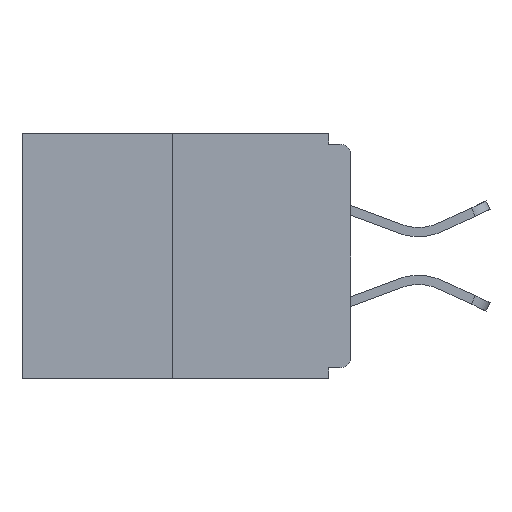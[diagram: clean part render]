
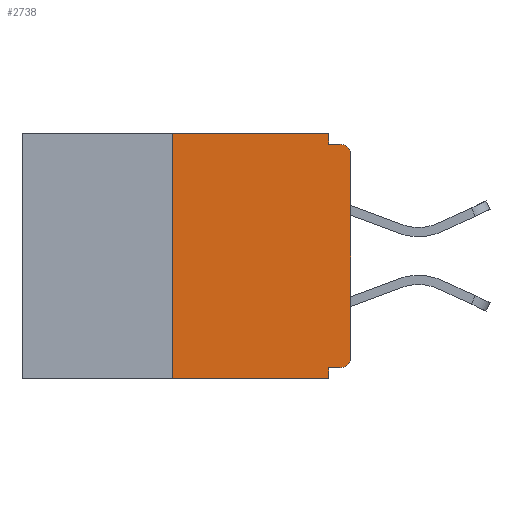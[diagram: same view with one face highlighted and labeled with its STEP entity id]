
A CAD part, left-side view. The second image highlights one B-rep face of the part: STEP entity #2738.
In plain terms, the highlighted planar face has unit normal (-1, 0, 0).
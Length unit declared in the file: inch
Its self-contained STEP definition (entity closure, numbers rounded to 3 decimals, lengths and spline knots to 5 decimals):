
#90 = DIRECTION ( 'NONE',  ( 0., 0., -1. ) ) ;
#414 = VECTOR ( 'NONE', #5295, 39.37008 ) ;
#443 = CARTESIAN_POINT ( 'NONE',  ( 0., 0.031, -0.015 ) ) ;
#765 = AXIS2_PLACEMENT_3D ( 'NONE', #9386, #5205, #12237 ) ;
#822 = CIRCLE ( 'NONE', #15565, 0.015 ) ;
#994 = CARTESIAN_POINT ( 'NONE',  ( 0., 0., -0.015 ) ) ;
#1052 = DIRECTION ( 'NONE',  ( 0., -1., 0. ) ) ;
#1104 = DIRECTION ( 'NONE',  ( 0., 1., 0. ) ) ;
#1154 = DIRECTION ( 'NONE',  ( 0., 0., 1. ) ) ;
#1769 = LINE ( 'NONE', #17970, #414 ) ;
#1825 = CIRCLE ( 'NONE', #765, 0.015 ) ;
#1953 = DIRECTION ( 'NONE',  ( 0., -1., 0. ) ) ;
#2083 = DIRECTION ( 'NONE',  ( 0., 0., -1. ) ) ;
#2545 = LINE ( 'NONE', #9125, #6310 ) ;
#2627 = LINE ( 'NONE', #17397, #12072 ) ;
#2664 = EDGE_CURVE ( 'NONE', #4280, #16776, #12251, .T. ) ;
#2697 = CARTESIAN_POINT ( 'NONE',  ( 0., 0.25, 0. ) ) ;
#2738 = ADVANCED_FACE ( 'NONE', ( #11829 ), #7510, .F. ) ;
#2756 = EDGE_CURVE ( 'NONE', #16776, #17188, #14868, .T. ) ;
#3808 = CARTESIAN_POINT ( 'NONE',  ( 0., 0., 0. ) ) ;
#4280 = VERTEX_POINT ( 'NONE', #15031 ) ;
#4948 = CARTESIAN_POINT ( 'NONE',  ( 0., 0.015, -0.015 ) ) ;
#5205 = DIRECTION ( 'NONE',  ( -1., 0., 0. ) ) ;
#5295 = DIRECTION ( 'NONE',  ( 0., -1., 0. ) ) ;
#5368 = ORIENTED_EDGE ( 'NONE', *, *, #13548, .F. ) ;
#5560 = CARTESIAN_POINT ( 'NONE',  ( 0., 0.25, -0.343 ) ) ;
#5586 = EDGE_LOOP ( 'NONE', ( #10900, #16993, #12227, #5658, #12666, #16436, #12895, #8664, #8403, #5368 ) ) ;
#5616 = VECTOR ( 'NONE', #6589, 39.37008 ) ;
#5658 = ORIENTED_EDGE ( 'NONE', *, *, #2756, .F. ) ;
#5759 = CARTESIAN_POINT ( 'NONE',  ( 0., 0.015, -0.313 ) ) ;
#6137 = EDGE_CURVE ( 'NONE', #11854, #13108, #1825, .T. ) ;
#6310 = VECTOR ( 'NONE', #2083, 39.37008 ) ;
#6589 = DIRECTION ( 'NONE',  ( 0., 0., 1. ) ) ;
#6967 = VECTOR ( 'NONE', #1104, 39.37008 ) ;
#7136 = VERTEX_POINT ( 'NONE', #443 ) ;
#7269 = DIRECTION ( 'NONE',  ( 0., 0., -1. ) ) ;
#7510 = PLANE ( 'NONE',  #13661 ) ;
#8403 = ORIENTED_EDGE ( 'NONE', *, *, #16284, .F. ) ;
#8664 = ORIENTED_EDGE ( 'NONE', *, *, #6137, .T. ) ;
#9125 = CARTESIAN_POINT ( 'NONE',  ( 0., 0.031, 0. ) ) ;
#9386 = CARTESIAN_POINT ( 'NONE',  ( 0., 0.015, -0.03 ) ) ;
#9465 = VECTOR ( 'NONE', #1052, 39.37008 ) ;
#9651 = CARTESIAN_POINT ( 'NONE',  ( 0., 0., -0.313 ) ) ;
#9660 = VECTOR ( 'NONE', #1154, 39.37008 ) ;
#9748 = VERTEX_POINT ( 'NONE', #9651 ) ;
#10900 = ORIENTED_EDGE ( 'NONE', *, *, #11726, .F. ) ;
#11543 = VERTEX_POINT ( 'NONE', #5560 ) ;
#11726 = EDGE_CURVE ( 'NONE', #17469, #14577, #2627, .T. ) ;
#11829 = FACE_OUTER_BOUND ( 'NONE', #5586, .T. ) ;
#11854 = VERTEX_POINT ( 'NONE', #12633 ) ;
#12072 = VECTOR ( 'NONE', #1953, 39.37008 ) ;
#12091 = CARTESIAN_POINT ( 'NONE',  ( 0., 0.25, 0. ) ) ;
#12227 = ORIENTED_EDGE ( 'NONE', *, *, #16669, .T. ) ;
#12237 = DIRECTION ( 'NONE',  ( 0., 0., -1. ) ) ;
#12251 = LINE ( 'NONE', #12402, #6967 ) ;
#12402 = CARTESIAN_POINT ( 'NONE',  ( 0., 0., -0.328 ) ) ;
#12543 = EDGE_CURVE ( 'NONE', #4280, #9748, #822, .T. ) ;
#12633 = CARTESIAN_POINT ( 'NONE',  ( 0., 0., -0.03 ) ) ;
#12666 = ORIENTED_EDGE ( 'NONE', *, *, #2664, .F. ) ;
#12732 = CARTESIAN_POINT ( 'NONE',  ( 0., 0.031, 0. ) ) ;
#12895 = ORIENTED_EDGE ( 'NONE', *, *, #13925, .T. ) ;
#12954 = DIRECTION ( 'NONE',  ( 1., 0., 0. ) ) ;
#13088 = CARTESIAN_POINT ( 'NONE',  ( 0., 0.031, -0.343 ) ) ;
#13108 = VERTEX_POINT ( 'NONE', #4948 ) ;
#13548 = EDGE_CURVE ( 'NONE', #14577, #7136, #2545, .T. ) ;
#13661 = AXIS2_PLACEMENT_3D ( 'NONE', #17242, #12954, #7269 ) ;
#13915 = CARTESIAN_POINT ( 'NONE',  ( 0., 0.031, -0.328 ) ) ;
#13925 = EDGE_CURVE ( 'NONE', #9748, #11854, #18180, .T. ) ;
#14063 = LINE ( 'NONE', #994, #9465 ) ;
#14577 = VERTEX_POINT ( 'NONE', #12732 ) ;
#14868 = LINE ( 'NONE', #13088, #15299 ) ;
#15031 = CARTESIAN_POINT ( 'NONE',  ( 0., 0.015, -0.328 ) ) ;
#15150 = CARTESIAN_POINT ( 'NONE',  ( 0., 0.031, -0.343 ) ) ;
#15299 = VECTOR ( 'NONE', #15778, 39.37008 ) ;
#15336 = LINE ( 'NONE', #12091, #9660 ) ;
#15565 = AXIS2_PLACEMENT_3D ( 'NONE', #5759, #18187, #90 ) ;
#15778 = DIRECTION ( 'NONE',  ( 0., 0., -1. ) ) ;
#16284 = EDGE_CURVE ( 'NONE', #7136, #13108, #14063, .T. ) ;
#16436 = ORIENTED_EDGE ( 'NONE', *, *, #12543, .T. ) ;
#16597 = EDGE_CURVE ( 'NONE', #11543, #17469, #15336, .T. ) ;
#16669 = EDGE_CURVE ( 'NONE', #11543, #17188, #1769, .T. ) ;
#16776 = VERTEX_POINT ( 'NONE', #13915 ) ;
#16993 = ORIENTED_EDGE ( 'NONE', *, *, #16597, .F. ) ;
#17188 = VERTEX_POINT ( 'NONE', #15150 ) ;
#17242 = CARTESIAN_POINT ( 'NONE',  ( 0., 0.46, 0. ) ) ;
#17397 = CARTESIAN_POINT ( 'NONE',  ( 0., 0.46, 0. ) ) ;
#17469 = VERTEX_POINT ( 'NONE', #2697 ) ;
#17970 = CARTESIAN_POINT ( 'NONE',  ( 0., 0.46, -0.343 ) ) ;
#18180 = LINE ( 'NONE', #3808, #5616 ) ;
#18187 = DIRECTION ( 'NONE',  ( -1., 0., 0. ) ) ;
